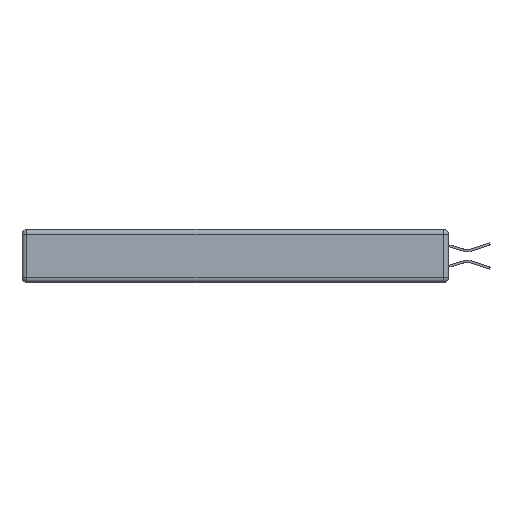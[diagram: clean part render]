
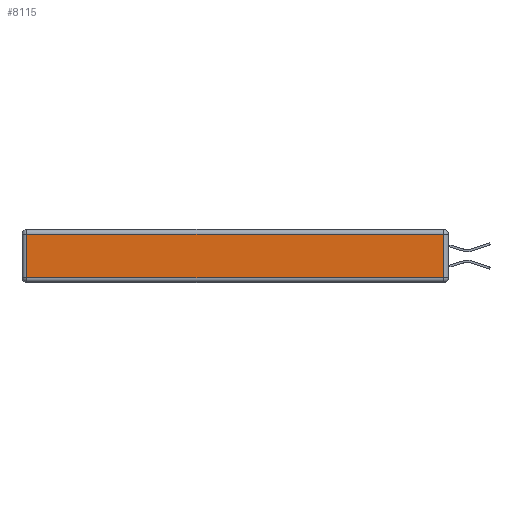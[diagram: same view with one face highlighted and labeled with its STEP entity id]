
A CAD part, left-side view. The second image highlights one B-rep face of the part: STEP entity #8115.
In plain terms, the highlighted planar face has unit normal (-1, 0, 0).
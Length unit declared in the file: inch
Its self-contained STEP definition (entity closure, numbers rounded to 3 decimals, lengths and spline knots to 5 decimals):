
#1194 = LINE ( 'NONE', #13703, #3585 ) ;
#1520 = CARTESIAN_POINT ( 'NONE',  ( 0., 2.72, -0.313 ) ) ;
#1871 = EDGE_LOOP ( 'NONE', ( #11928, #14065, #7179, #8381 ) ) ;
#3049 = VERTEX_POINT ( 'NONE', #12682 ) ;
#3585 = VECTOR ( 'NONE', #11363, 39.37008 ) ;
#4307 = VECTOR ( 'NONE', #11629, 39.37008 ) ;
#5269 = DIRECTION ( 'NONE',  ( 0., 0., 1. ) ) ;
#5906 = LINE ( 'NONE', #13944, #9945 ) ;
#6207 = LINE ( 'NONE', #13351, #8598 ) ;
#6675 = EDGE_CURVE ( 'NONE', #11032, #3049, #9826, .T. ) ;
#6722 = EDGE_CURVE ( 'NONE', #8065, #12182, #5906, .T. ) ;
#6889 = DIRECTION ( 'NONE',  ( 0., 0., -1. ) ) ;
#7179 = ORIENTED_EDGE ( 'NONE', *, *, #8665, .T. ) ;
#7217 = CARTESIAN_POINT ( 'NONE',  ( 0., 0., -0.343 ) ) ;
#8065 = VERTEX_POINT ( 'NONE', #13063 ) ;
#8115 = ADVANCED_FACE ( 'NONE', ( #13004 ), #8558, .T. ) ;
#8381 = ORIENTED_EDGE ( 'NONE', *, *, #6722, .T. ) ;
#8558 = PLANE ( 'NONE',  #13472 ) ;
#8598 = VECTOR ( 'NONE', #9865, 39.37008 ) ;
#8665 = EDGE_CURVE ( 'NONE', #3049, #8065, #6207, .T. ) ;
#9140 = EDGE_CURVE ( 'NONE', #12182, #11032, #1194, .T. ) ;
#9826 = LINE ( 'NONE', #12747, #4307 ) ;
#9865 = DIRECTION ( 'NONE',  ( 0., 1., 0. ) ) ;
#9945 = VECTOR ( 'NONE', #6889, 39.37008 ) ;
#11032 = VERTEX_POINT ( 'NONE', #14455 ) ;
#11363 = DIRECTION ( 'NONE',  ( 0., -1., 0. ) ) ;
#11629 = DIRECTION ( 'NONE',  ( 0., 0., 1. ) ) ;
#11928 = ORIENTED_EDGE ( 'NONE', *, *, #9140, .T. ) ;
#12182 = VERTEX_POINT ( 'NONE', #1520 ) ;
#12309 = DIRECTION ( 'NONE',  ( -1., 0., 0. ) ) ;
#12682 = CARTESIAN_POINT ( 'NONE',  ( 0., 0.03, -0.03 ) ) ;
#12747 = CARTESIAN_POINT ( 'NONE',  ( 0., 0.03, -0.343 ) ) ;
#13004 = FACE_OUTER_BOUND ( 'NONE', #1871, .T. ) ;
#13063 = CARTESIAN_POINT ( 'NONE',  ( 0., 2.72, -0.03 ) ) ;
#13351 = CARTESIAN_POINT ( 'NONE',  ( 0., 2.75, -0.03 ) ) ;
#13472 = AXIS2_PLACEMENT_3D ( 'NONE', #7217, #12309, #5269 ) ;
#13703 = CARTESIAN_POINT ( 'NONE',  ( 0., 0., -0.313 ) ) ;
#13944 = CARTESIAN_POINT ( 'NONE',  ( 0., 2.72, -0.343 ) ) ;
#14065 = ORIENTED_EDGE ( 'NONE', *, *, #6675, .T. ) ;
#14455 = CARTESIAN_POINT ( 'NONE',  ( 0., 0.03, -0.313 ) ) ;
